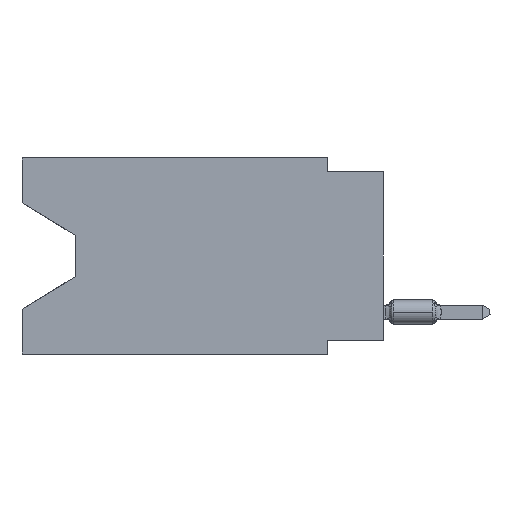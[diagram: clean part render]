
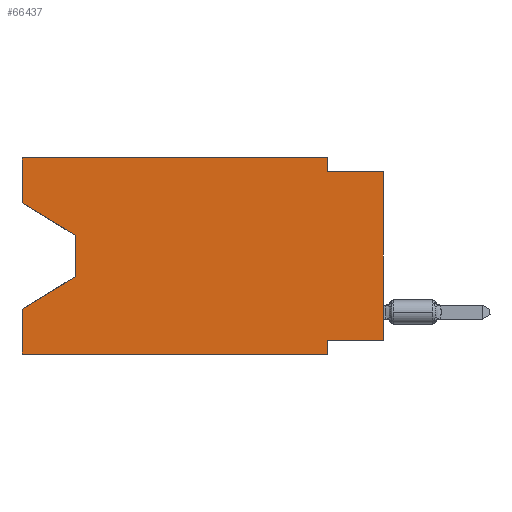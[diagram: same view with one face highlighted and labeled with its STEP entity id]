
A CAD part, left-side view. The second image highlights one B-rep face of the part: STEP entity #66437.
In plain terms, the highlighted planar face has unit normal (-1, 0, 0).
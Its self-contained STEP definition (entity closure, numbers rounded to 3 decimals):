
#640 = EDGE_CURVE ( 'NONE', #5207, #63583, #49058, .T. ) ;
#2345 = DIRECTION ( 'NONE',  ( 0., 1., 0. ) ) ;
#5207 = VERTEX_POINT ( 'NONE', #26155 ) ;
#5650 = ORIENTED_EDGE ( 'NONE', *, *, #96257, .T. ) ;
#7328 = CARTESIAN_POINT ( 'NONE',  ( 0., 16.383, -6.852 ) ) ;
#8406 = CARTESIAN_POINT ( 'NONE',  ( 0., 16.383, -2.038 ) ) ;
#9801 = CARTESIAN_POINT ( 'NONE',  ( 0., 13.97, -5.385 ) ) ;
#14191 = DIRECTION ( 'NONE',  ( 0., 0., 1. ) ) ;
#14640 = ORIENTED_EDGE ( 'NONE', *, *, #93267, .T. ) ;
#15509 = VERTEX_POINT ( 'NONE', #68163 ) ;
#19595 = VECTOR ( 'NONE', #2345, 1000. ) ;
#20056 = CARTESIAN_POINT ( 'NONE',  ( 0., 16.383, 0. ) ) ;
#21410 = CARTESIAN_POINT ( 'NONE',  ( 0., 13.97, -5.385 ) ) ;
#22285 = VECTOR ( 'NONE', #42949, 1000. ) ;
#22835 = DIRECTION ( 'NONE',  ( 0., 0., 1. ) ) ;
#24775 = CARTESIAN_POINT ( 'NONE',  ( 0., 16.383, 0. ) ) ;
#25299 = EDGE_LOOP ( 'NONE', ( #91083, #14640, #38328, #106115, #5650, #106590, #89346, #105101, #53591, #41344, #71168, #60355 ) ) ;
#25840 = EDGE_CURVE ( 'NONE', #63583, #36317, #80924, .T. ) ;
#26155 = CARTESIAN_POINT ( 'NONE',  ( 0., 2.54, 0. ) ) ;
#27911 = LINE ( 'NONE', #59975, #40150 ) ;
#28558 = CARTESIAN_POINT ( 'NONE',  ( 0., 2.54, -0.635 ) ) ;
#29123 = VERTEX_POINT ( 'NONE', #7328 ) ;
#29214 = CARTESIAN_POINT ( 'NONE',  ( 0., 2.54, -8.89 ) ) ;
#34221 = CARTESIAN_POINT ( 'NONE',  ( 0., 16.383, -2.038 ) ) ;
#34529 = VERTEX_POINT ( 'NONE', #24775 ) ;
#36317 = VERTEX_POINT ( 'NONE', #48439 ) ;
#38140 = EDGE_CURVE ( 'NONE', #34529, #5207, #38299, .T. ) ;
#38299 = LINE ( 'NONE', #54563, #60429 ) ;
#38328 = ORIENTED_EDGE ( 'NONE', *, *, #102696, .T. ) ;
#39487 = VERTEX_POINT ( 'NONE', #8406 ) ;
#40150 = VECTOR ( 'NONE', #83821, 1000. ) ;
#40523 = VERTEX_POINT ( 'NONE', #29214 ) ;
#40686 = VECTOR ( 'NONE', #72429, 1000. ) ;
#41344 = ORIENTED_EDGE ( 'NONE', *, *, #640, .F. ) ;
#41802 = LINE ( 'NONE', #34221, #100124 ) ;
#42949 = DIRECTION ( 'NONE',  ( 0., 0., 1. ) ) ;
#43566 = LINE ( 'NONE', #101575, #19595 ) ;
#45025 = DIRECTION ( 'NONE',  ( 1., 0., 0. ) ) ;
#48341 = CARTESIAN_POINT ( 'NONE',  ( 0., 16.383, 0. ) ) ;
#48439 = CARTESIAN_POINT ( 'NONE',  ( 0., 0., -0.635 ) ) ;
#48525 = CARTESIAN_POINT ( 'NONE',  ( 0., 2.54, 0. ) ) ;
#49058 = LINE ( 'NONE', #48525, #40686 ) ;
#51528 = VECTOR ( 'NONE', #14191, 1000. ) ;
#53591 = ORIENTED_EDGE ( 'NONE', *, *, #25840, .F. ) ;
#53606 = EDGE_CURVE ( 'NONE', #102657, #40523, #105591, .T. ) ;
#53814 = CARTESIAN_POINT ( 'NONE',  ( 0., 0., 0. ) ) ;
#54100 = DIRECTION ( 'NONE',  ( 0., 0., -1. ) ) ;
#54563 = CARTESIAN_POINT ( 'NONE',  ( 0., 16.383, 0. ) ) ;
#59975 = CARTESIAN_POINT ( 'NONE',  ( 0., 16.383, -8.89 ) ) ;
#60355 = ORIENTED_EDGE ( 'NONE', *, *, #106165, .F. ) ;
#60429 = VECTOR ( 'NONE', #71922, 1000. ) ;
#60738 = DIRECTION ( 'NONE',  ( 0., 0., -1. ) ) ;
#63114 = VECTOR ( 'NONE', #54100, 1000. ) ;
#63583 = VERTEX_POINT ( 'NONE', #28558 ) ;
#64403 = CARTESIAN_POINT ( 'NONE',  ( 0., 2.54, -8.89 ) ) ;
#66437 = ADVANCED_FACE ( 'NONE', ( #69441 ), #94375, .F. ) ;
#66611 = VERTEX_POINT ( 'NONE', #90520 ) ;
#66944 = VECTOR ( 'NONE', #97187, 1000. ) ;
#68163 = CARTESIAN_POINT ( 'NONE',  ( 0., 16.383, -8.89 ) ) ;
#68679 = EDGE_CURVE ( 'NONE', #15509, #29123, #78760, .T. ) ;
#69441 = FACE_OUTER_BOUND ( 'NONE', #25299, .T. ) ;
#69501 = CARTESIAN_POINT ( 'NONE',  ( 0., 16.383, 0. ) ) ;
#71168 = ORIENTED_EDGE ( 'NONE', *, *, #38140, .F. ) ;
#71343 = DIRECTION ( 'NONE',  ( 0., 0.855, -0.519 ) ) ;
#71552 = VECTOR ( 'NONE', #22835, 1000. ) ;
#71882 = CARTESIAN_POINT ( 'NONE',  ( 0., 2.54, -8.255 ) ) ;
#71922 = DIRECTION ( 'NONE',  ( 0., -1., 0. ) ) ;
#72429 = DIRECTION ( 'NONE',  ( 0., 0., -1. ) ) ;
#74895 = DIRECTION ( 'NONE',  ( 0., -0.855, -0.519 ) ) ;
#76044 = EDGE_CURVE ( 'NONE', #66611, #36317, #78787, .T. ) ;
#76726 = EDGE_CURVE ( 'NONE', #39487, #87475, #41802, .T. ) ;
#77204 = CARTESIAN_POINT ( 'NONE',  ( 0., 13.97, -3.505 ) ) ;
#77973 = VERTEX_POINT ( 'NONE', #9801 ) ;
#78119 = DIRECTION ( 'NONE',  ( 0., 0., -1. ) ) ;
#78760 = LINE ( 'NONE', #48341, #71552 ) ;
#78787 = LINE ( 'NONE', #53814, #51528 ) ;
#80841 = EDGE_CURVE ( 'NONE', #66611, #102657, #43566, .T. ) ;
#80924 = LINE ( 'NONE', #105838, #66944 ) ;
#81560 = VECTOR ( 'NONE', #60738, 1000. ) ;
#83154 = AXIS2_PLACEMENT_3D ( 'NONE', #20056, #45025, #78119 ) ;
#83821 = DIRECTION ( 'NONE',  ( 0., -1., 0. ) ) ;
#87475 = VERTEX_POINT ( 'NONE', #77204 ) ;
#88683 = LINE ( 'NONE', #21410, #94466 ) ;
#89346 = ORIENTED_EDGE ( 'NONE', *, *, #80841, .F. ) ;
#90520 = CARTESIAN_POINT ( 'NONE',  ( 0., 0., -8.255 ) ) ;
#91083 = ORIENTED_EDGE ( 'NONE', *, *, #76726, .T. ) ;
#93267 = EDGE_CURVE ( 'NONE', #87475, #77973, #93275, .T. ) ;
#93275 = LINE ( 'NONE', #99785, #81560 ) ;
#94375 = PLANE ( 'NONE',  #83154 ) ;
#94437 = LINE ( 'NONE', #69501, #22285 ) ;
#94466 = VECTOR ( 'NONE', #71343, 1000. ) ;
#96257 = EDGE_CURVE ( 'NONE', #15509, #40523, #27911, .T. ) ;
#97187 = DIRECTION ( 'NONE',  ( 0., -1., 0. ) ) ;
#99785 = CARTESIAN_POINT ( 'NONE',  ( 0., 13.97, -3.505 ) ) ;
#100124 = VECTOR ( 'NONE', #74895, 1000. ) ;
#101575 = CARTESIAN_POINT ( 'NONE',  ( 0., 0., -8.255 ) ) ;
#102657 = VERTEX_POINT ( 'NONE', #71882 ) ;
#102696 = EDGE_CURVE ( 'NONE', #77973, #29123, #88683, .T. ) ;
#105101 = ORIENTED_EDGE ( 'NONE', *, *, #76044, .T. ) ;
#105591 = LINE ( 'NONE', #64403, #63114 ) ;
#105838 = CARTESIAN_POINT ( 'NONE',  ( 0., 0., -0.635 ) ) ;
#106115 = ORIENTED_EDGE ( 'NONE', *, *, #68679, .F. ) ;
#106165 = EDGE_CURVE ( 'NONE', #39487, #34529, #94437, .T. ) ;
#106590 = ORIENTED_EDGE ( 'NONE', *, *, #53606, .F. ) ;
